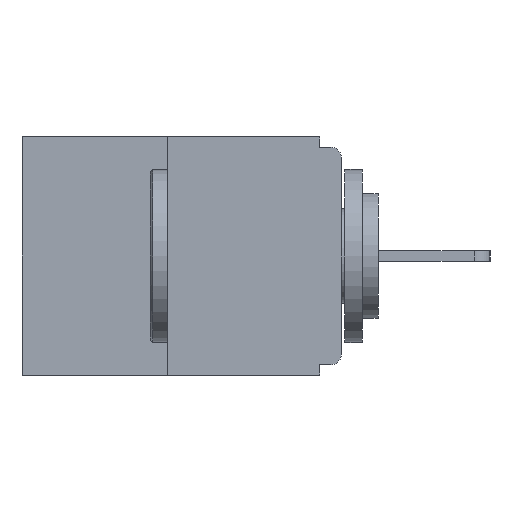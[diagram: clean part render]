
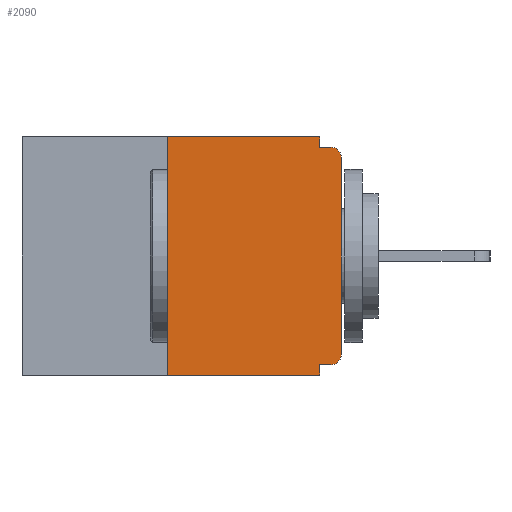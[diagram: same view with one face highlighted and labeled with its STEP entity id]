
A CAD part, left-side view. The second image highlights one B-rep face of the part: STEP entity #2090.
In plain terms, the highlighted planar face has unit normal (-1, 0, 0).
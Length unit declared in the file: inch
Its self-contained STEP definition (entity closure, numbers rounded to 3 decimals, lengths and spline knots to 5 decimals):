
#149 = VERTEX_POINT ( 'NONE', #8867 ) ;
#192 = AXIS2_PLACEMENT_3D ( 'NONE', #14089, #14061, #13979 ) ;
#223 = FACE_OUTER_BOUND ( 'NONE', #15271, .T. ) ;
#1255 = EDGE_CURVE ( 'NONE', #149, #4815, #3603, .T. ) ;
#1349 = DIRECTION ( 'NONE',  ( 0., -1., 0. ) ) ;
#1391 = CIRCLE ( 'NONE', #14765, 0.015 ) ;
#1399 = EDGE_CURVE ( 'NONE', #17963, #1853, #10598, .T. ) ;
#1429 = CARTESIAN_POINT ( 'NONE',  ( 0., 0.25, 0. ) ) ;
#1853 = VERTEX_POINT ( 'NONE', #8643 ) ;
#2090 = ADVANCED_FACE ( 'NONE', ( #223 ), #20199, .F. ) ;
#2433 = ORIENTED_EDGE ( 'NONE', *, *, #11496, .F. ) ;
#2470 = CARTESIAN_POINT ( 'NONE',  ( 0., 0., -0.313 ) ) ;
#3458 = ORIENTED_EDGE ( 'NONE', *, *, #7571, .T. ) ;
#3603 = LINE ( 'NONE', #11459, #12911 ) ;
#4171 = VERTEX_POINT ( 'NONE', #7765 ) ;
#4745 = EDGE_CURVE ( 'NONE', #22809, #10888, #12143, .T. ) ;
#4815 = VERTEX_POINT ( 'NONE', #11930 ) ;
#6566 = LINE ( 'NONE', #22007, #15677 ) ;
#6633 = DIRECTION ( 'NONE',  ( 0., 0., -1. ) ) ;
#6638 = DIRECTION ( 'NONE',  ( 1., 0., 0. ) ) ;
#6743 = ORIENTED_EDGE ( 'NONE', *, *, #8023, .T. ) ;
#7571 = EDGE_CURVE ( 'NONE', #149, #19232, #21138, .T. ) ;
#7584 = AXIS2_PLACEMENT_3D ( 'NONE', #23341, #6638, #6633 ) ;
#7765 = CARTESIAN_POINT ( 'NONE',  ( 0., 0.031, 0. ) ) ;
#8023 = EDGE_CURVE ( 'NONE', #12454, #1853, #1391, .T. ) ;
#8643 = CARTESIAN_POINT ( 'NONE',  ( 0., 0.015, -0.015 ) ) ;
#8867 = CARTESIAN_POINT ( 'NONE',  ( 0., 0.015, -0.328 ) ) ;
#8951 = CARTESIAN_POINT ( 'NONE',  ( 0., 0.25, 0. ) ) ;
#9343 = CARTESIAN_POINT ( 'NONE',  ( 0., 0.25, -0.343 ) ) ;
#9484 = VECTOR ( 'NONE', #1349, 39.37008 ) ;
#10016 = VECTOR ( 'NONE', #16765, 39.37008 ) ;
#10598 = LINE ( 'NONE', #20847, #10016 ) ;
#10754 = DIRECTION ( 'NONE',  ( 0., 1., 0. ) ) ;
#10868 = DIRECTION ( 'NONE',  ( -1., 0., 0. ) ) ;
#10888 = VERTEX_POINT ( 'NONE', #20416 ) ;
#10918 = DIRECTION ( 'NONE',  ( 0., 0., -1. ) ) ;
#10975 = CARTESIAN_POINT ( 'NONE',  ( 0., 0.015, -0.03 ) ) ;
#11122 = CARTESIAN_POINT ( 'NONE',  ( 0., 0.031, -0.343 ) ) ;
#11217 = ORIENTED_EDGE ( 'NONE', *, *, #13456, .F. ) ;
#11459 = CARTESIAN_POINT ( 'NONE',  ( 0., 0., -0.328 ) ) ;
#11496 = EDGE_CURVE ( 'NONE', #4171, #17963, #6566, .T. ) ;
#11775 = ORIENTED_EDGE ( 'NONE', *, *, #1399, .F. ) ;
#11781 = EDGE_CURVE ( 'NONE', #11828, #4171, #19916, .T. ) ;
#11796 = ORIENTED_EDGE ( 'NONE', *, *, #1255, .F. ) ;
#11828 = VERTEX_POINT ( 'NONE', #1429 ) ;
#11930 = CARTESIAN_POINT ( 'NONE',  ( 0., 0.031, -0.328 ) ) ;
#12070 = DIRECTION ( 'NONE',  ( 0., 0., 1. ) ) ;
#12143 = LINE ( 'NONE', #17765, #20729 ) ;
#12454 = VERTEX_POINT ( 'NONE', #13019 ) ;
#12911 = VECTOR ( 'NONE', #10754, 39.37008 ) ;
#13019 = CARTESIAN_POINT ( 'NONE',  ( 0., 0., -0.03 ) ) ;
#13456 = EDGE_CURVE ( 'NONE', #22809, #11828, #16401, .T. ) ;
#13519 = DIRECTION ( 'NONE',  ( 0., 0., -1. ) ) ;
#13636 = LINE ( 'NONE', #11122, #18186 ) ;
#13979 = DIRECTION ( 'NONE',  ( 0., 0., -1. ) ) ;
#14061 = DIRECTION ( 'NONE',  ( -1., 0., 0. ) ) ;
#14089 = CARTESIAN_POINT ( 'NONE',  ( 0., 0.015, -0.313 ) ) ;
#14561 = DIRECTION ( 'NONE',  ( 0., 0., 1. ) ) ;
#14765 = AXIS2_PLACEMENT_3D ( 'NONE', #10975, #10868, #10918 ) ;
#15271 = EDGE_LOOP ( 'NONE', ( #20766, #11217, #18395, #23313, #11796, #3458, #18588, #6743, #11775, #2433 ) ) ;
#15372 = DIRECTION ( 'NONE',  ( 0., -1., 0. ) ) ;
#15677 = VECTOR ( 'NONE', #13519, 39.37008 ) ;
#16096 = CARTESIAN_POINT ( 'NONE',  ( 0., 0.46, 0. ) ) ;
#16401 = LINE ( 'NONE', #8951, #20356 ) ;
#16493 = CARTESIAN_POINT ( 'NONE',  ( 0., 0.031, -0.015 ) ) ;
#16765 = DIRECTION ( 'NONE',  ( 0., -1., 0. ) ) ;
#17234 = CARTESIAN_POINT ( 'NONE',  ( 0., 0., 0. ) ) ;
#17765 = CARTESIAN_POINT ( 'NONE',  ( 0., 0.46, -0.343 ) ) ;
#17963 = VERTEX_POINT ( 'NONE', #16493 ) ;
#18186 = VECTOR ( 'NONE', #23179, 39.37008 ) ;
#18395 = ORIENTED_EDGE ( 'NONE', *, *, #4745, .T. ) ;
#18472 = EDGE_CURVE ( 'NONE', #4815, #10888, #13636, .T. ) ;
#18588 = ORIENTED_EDGE ( 'NONE', *, *, #19313, .T. ) ;
#18676 = LINE ( 'NONE', #17234, #22645 ) ;
#19232 = VERTEX_POINT ( 'NONE', #2470 ) ;
#19313 = EDGE_CURVE ( 'NONE', #19232, #12454, #18676, .T. ) ;
#19916 = LINE ( 'NONE', #16096, #9484 ) ;
#20199 = PLANE ( 'NONE',  #7584 ) ;
#20356 = VECTOR ( 'NONE', #14561, 39.37008 ) ;
#20416 = CARTESIAN_POINT ( 'NONE',  ( 0., 0.031, -0.343 ) ) ;
#20729 = VECTOR ( 'NONE', #15372, 39.37008 ) ;
#20766 = ORIENTED_EDGE ( 'NONE', *, *, #11781, .F. ) ;
#20847 = CARTESIAN_POINT ( 'NONE',  ( 0., 0., -0.015 ) ) ;
#21138 = CIRCLE ( 'NONE', #192, 0.015 ) ;
#22007 = CARTESIAN_POINT ( 'NONE',  ( 0., 0.031, 0. ) ) ;
#22645 = VECTOR ( 'NONE', #12070, 39.37008 ) ;
#22809 = VERTEX_POINT ( 'NONE', #9343 ) ;
#23179 = DIRECTION ( 'NONE',  ( 0., 0., -1. ) ) ;
#23313 = ORIENTED_EDGE ( 'NONE', *, *, #18472, .F. ) ;
#23341 = CARTESIAN_POINT ( 'NONE',  ( 0., 0.46, 0. ) ) ;
